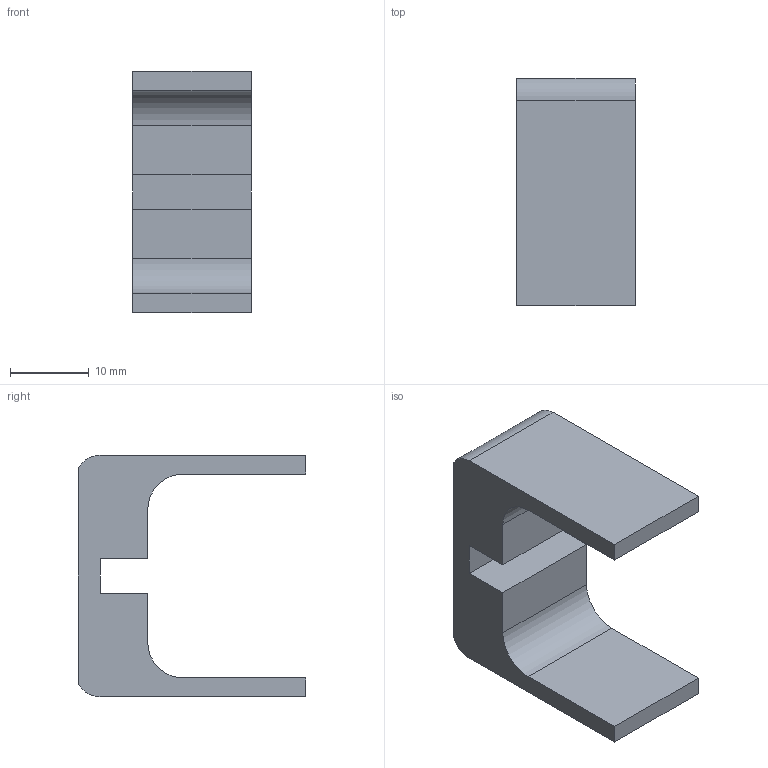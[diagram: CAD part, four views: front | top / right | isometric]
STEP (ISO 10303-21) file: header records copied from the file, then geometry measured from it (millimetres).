
FILE_DESCRIPTION(/* description */ (''),/* implementation_level */ '2;1');
FILE_NAME(/* name */ 'GL_sight_alignment_tool.step',/* time_stamp */ '2022-01-11T21:09:48-05:00',/* author */ (''),/* organization */ (''),/* preprocessor_version */ 'ST-DEVELOPER v18.1',/* originating_system */ 'Autodesk Translation Framework v10.10.0.1391',/* authorisation */ '');
FILE_SCHEMA (('AUTOMOTIVE_DESIGN { 1 0 10303 214 3 1 1 }'));
Length unit declared in the file: millimetre
Products named in the file (1): Snow-G-Sight
Bounding box: 15 x 28.8 x 30.6 mm (x, y, z)
Volume: 5111.4 mm3; surface area: 3453 mm2
Topology: 1 solids, 1 shells, 330 faces, 954 edges, 636 vertices
Faces by surface type: plane 176, bspline 150, cylinder 4
Entity records: 11183 total; most frequent: CARTESIAN_POINT 3775, ORIENTED_EDGE 1908, DIRECTION 1104, EDGE_CURVE 954, LINE 646, VECTOR 646, VERTEX_POINT 636, EDGE_LOOP 340
